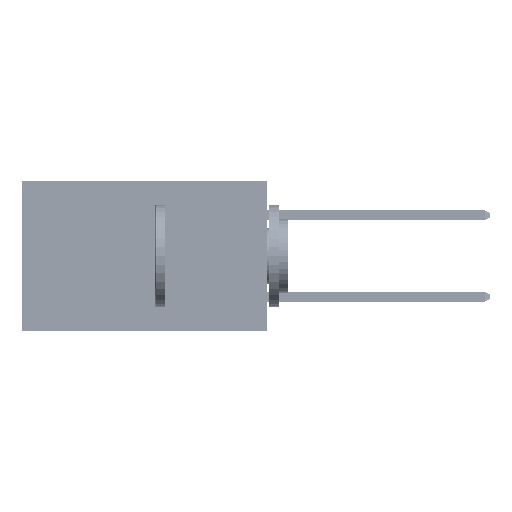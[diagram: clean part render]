
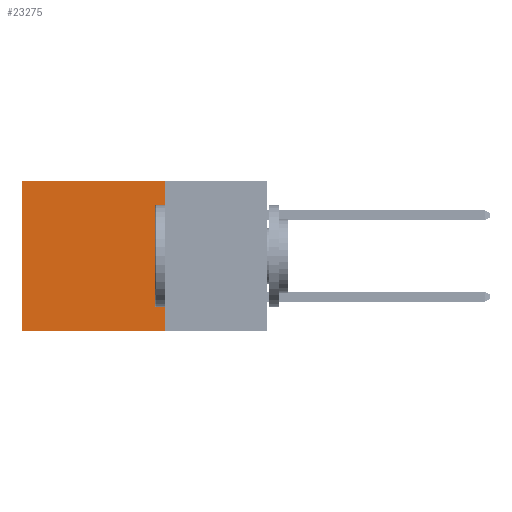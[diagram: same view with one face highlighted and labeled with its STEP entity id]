
A CAD part, left-side view. The second image highlights one B-rep face of the part: STEP entity #23275.
In plain terms, the highlighted planar face has unit normal (-1, 0, 0).
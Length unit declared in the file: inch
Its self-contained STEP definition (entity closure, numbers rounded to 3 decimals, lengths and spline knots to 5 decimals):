
#1128 = LINE ( 'NONE', #41094, #30039 ) ;
#2064 = CARTESIAN_POINT ( 'NONE',  ( 0.2875, 0.25, 0. ) ) ;
#2479 = PLANE ( 'NONE',  #4612 ) ;
#3898 = ORIENTED_EDGE ( 'NONE', *, *, #44785, .F. ) ;
#4612 = AXIS2_PLACEMENT_3D ( 'NONE', #14876, #10584, #30538 ) ;
#5181 = VERTEX_POINT ( 'NONE', #2064 ) ;
#5562 = VECTOR ( 'NONE', #17210, 39.37008 ) ;
#5913 = VERTEX_POINT ( 'NONE', #18964 ) ;
#10584 = DIRECTION ( 'NONE',  ( 1., 0., 0. ) ) ;
#10967 = LINE ( 'NONE', #43150, #50150 ) ;
#12050 = CARTESIAN_POINT ( 'NONE',  ( 0.2875, 0.25, -0.37 ) ) ;
#14876 = CARTESIAN_POINT ( 'NONE',  ( 0.2875, 0.25, 0. ) ) ;
#15428 = FACE_OUTER_BOUND ( 'NONE', #27121, .T. ) ;
#17073 = LINE ( 'NONE', #50052, #5562 ) ;
#17210 = DIRECTION ( 'NONE',  ( 0., 0., -1. ) ) ;
#18964 = CARTESIAN_POINT ( 'NONE',  ( 0.2875, 0.6, -0.37 ) ) ;
#19167 = VERTEX_POINT ( 'NONE', #12050 ) ;
#23275 = ADVANCED_FACE ( 'NONE', ( #15428 ), #2479, .F. ) ;
#26564 = EDGE_CURVE ( 'NONE', #5181, #19167, #17073, .T. ) ;
#27121 = EDGE_LOOP ( 'NONE', ( #41945, #3898, #49137, #35768 ) ) ;
#28045 = LINE ( 'NONE', #32670, #35135 ) ;
#30039 = VECTOR ( 'NONE', #53074, 39.37008 ) ;
#30538 = DIRECTION ( 'NONE',  ( 0., 0., -1. ) ) ;
#32670 = CARTESIAN_POINT ( 'NONE',  ( 0.2875, 0.25, 0. ) ) ;
#33100 = CARTESIAN_POINT ( 'NONE',  ( 0.2875, 0.6, 0. ) ) ;
#34384 = VERTEX_POINT ( 'NONE', #33100 ) ;
#34959 = EDGE_CURVE ( 'NONE', #34384, #5913, #1128, .T. ) ;
#35135 = VECTOR ( 'NONE', #40737, 39.37008 ) ;
#35768 = ORIENTED_EDGE ( 'NONE', *, *, #47587, .T. ) ;
#40737 = DIRECTION ( 'NONE',  ( 0., 1., 0. ) ) ;
#41094 = CARTESIAN_POINT ( 'NONE',  ( 0.2875, 0.6, 0. ) ) ;
#41945 = ORIENTED_EDGE ( 'NONE', *, *, #34959, .T. ) ;
#42631 = DIRECTION ( 'NONE',  ( 0., 1., 0. ) ) ;
#43150 = CARTESIAN_POINT ( 'NONE',  ( 0.2875, 0.25, -0.37 ) ) ;
#44785 = EDGE_CURVE ( 'NONE', #19167, #5913, #10967, .T. ) ;
#47587 = EDGE_CURVE ( 'NONE', #5181, #34384, #28045, .T. ) ;
#49137 = ORIENTED_EDGE ( 'NONE', *, *, #26564, .F. ) ;
#50052 = CARTESIAN_POINT ( 'NONE',  ( 0.2875, 0.25, 0. ) ) ;
#50150 = VECTOR ( 'NONE', #42631, 39.37008 ) ;
#53074 = DIRECTION ( 'NONE',  ( 0., 0., -1. ) ) ;
